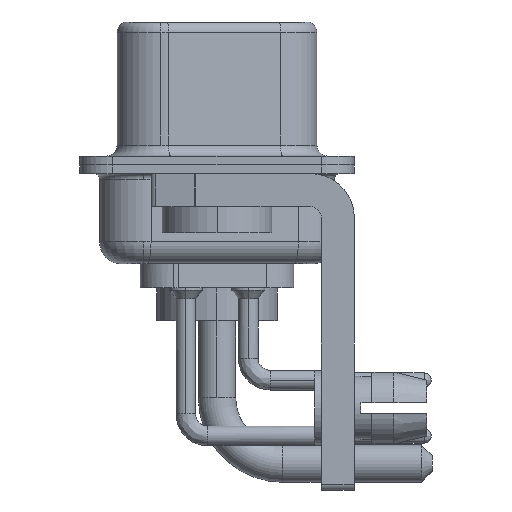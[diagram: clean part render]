
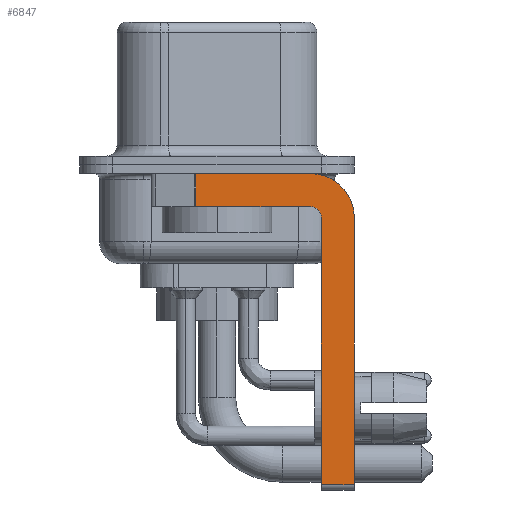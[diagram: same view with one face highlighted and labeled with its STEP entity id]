
A CAD part, left-side view. The second image highlights one B-rep face of the part: STEP entity #6847.
In plain terms, the highlighted planar face has unit normal (-1, 0, 0).
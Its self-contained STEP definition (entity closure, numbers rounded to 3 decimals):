
#1237 = CARTESIAN_POINT ( 'NONE',  ( -2.9, -4.25, -2.4 ) ) ;
#2401 = CIRCLE ( 'NONE', #5590, 2. ) ;
#2518 = VERTEX_POINT ( 'NONE', #2725 ) ;
#2519 = DIRECTION ( 'NONE',  ( 1., 0., 0. ) ) ;
#2725 = CARTESIAN_POINT ( 'NONE',  ( -2.9, -6.25, -14.55 ) ) ;
#2909 = CARTESIAN_POINT ( 'NONE',  ( -2.9, -4.75, -2.4 ) ) ;
#3019 = CARTESIAN_POINT ( 'NONE',  ( -2.9, -4.75, -14.8 ) ) ;
#3163 = ORIENTED_EDGE ( 'NONE', *, *, #10574, .F. ) ;
#3232 = EDGE_LOOP ( 'NONE', ( #4987, #20058, #3163, #21788, #18680, #17428, #16876, #21166 ) ) ;
#3481 = CARTESIAN_POINT ( 'NONE',  ( -2.9, -4.25, -2.4 ) ) ;
#4480 = VECTOR ( 'NONE', #5663, 1000. ) ;
#4587 = DIRECTION ( 'NONE',  ( 0., 0., -1. ) ) ;
#4697 = LINE ( 'NONE', #15106, #12434 ) ;
#4965 = CARTESIAN_POINT ( 'NONE',  ( -2.9, -6.25, -2.4 ) ) ;
#4987 = ORIENTED_EDGE ( 'NONE', *, *, #9422, .F. ) ;
#5192 = LINE ( 'NONE', #11982, #18535 ) ;
#5563 = VERTEX_POINT ( 'NONE', #15872 ) ;
#5590 = AXIS2_PLACEMENT_3D ( 'NONE', #3481, #11929, #20415 ) ;
#5663 = DIRECTION ( 'NONE',  ( 0., 0., -1. ) ) ;
#6539 = VECTOR ( 'NONE', #16546, 1000. ) ;
#6847 = ADVANCED_FACE ( 'NONE', ( #11187 ), #12530, .F. ) ;
#7184 = VERTEX_POINT ( 'NONE', #10415 ) ;
#7391 = AXIS2_PLACEMENT_3D ( 'NONE', #1237, #14770, #19745 ) ;
#8220 = VERTEX_POINT ( 'NONE', #19374 ) ;
#8953 = CARTESIAN_POINT ( 'NONE',  ( -2.9, 0.978, -1.9 ) ) ;
#9261 = CARTESIAN_POINT ( 'NONE',  ( -2.9, 3., -0.4 ) ) ;
#9422 = EDGE_CURVE ( 'NONE', #5563, #17456, #12898, .T. ) ;
#9888 = EDGE_CURVE ( 'NONE', #16541, #2518, #16301, .T. ) ;
#10415 = CARTESIAN_POINT ( 'NONE',  ( -2.9, -4.75, -14.55 ) ) ;
#10536 = VECTOR ( 'NONE', #11935, 1000. ) ;
#10550 = VECTOR ( 'NONE', #16099, 1000. ) ;
#10574 = EDGE_CURVE ( 'NONE', #8220, #13044, #18664, .T. ) ;
#11187 = FACE_OUTER_BOUND ( 'NONE', #3232, .T. ) ;
#11207 = CARTESIAN_POINT ( 'NONE',  ( -2.9, -6.25, -2.4 ) ) ;
#11294 = EDGE_CURVE ( 'NONE', #17456, #16541, #2401, .T. ) ;
#11659 = EDGE_CURVE ( 'NONE', #18870, #8220, #16226, .T. ) ;
#11929 = DIRECTION ( 'NONE',  ( 1., 0., 0. ) ) ;
#11935 = DIRECTION ( 'NONE',  ( 0., 1., 0. ) ) ;
#11982 = CARTESIAN_POINT ( 'NONE',  ( -2.9, -4.25, -14.55 ) ) ;
#12434 = VECTOR ( 'NONE', #4587, 1000. ) ;
#12530 = PLANE ( 'NONE',  #17651 ) ;
#12898 = LINE ( 'NONE', #9261, #10550 ) ;
#13044 = VERTEX_POINT ( 'NONE', #8953 ) ;
#13380 = CARTESIAN_POINT ( 'NONE',  ( -2.9, -4.25, -1.9 ) ) ;
#13950 = EDGE_CURVE ( 'NONE', #5563, #13044, #4697, .T. ) ;
#14770 = DIRECTION ( 'NONE',  ( -1., 0., 0. ) ) ;
#15106 = CARTESIAN_POINT ( 'NONE',  ( -2.9, 0.978, -1.9 ) ) ;
#15872 = CARTESIAN_POINT ( 'NONE',  ( -2.9, 0.978, -0.4 ) ) ;
#16099 = DIRECTION ( 'NONE',  ( 0., -1., 0. ) ) ;
#16128 = EDGE_CURVE ( 'NONE', #7184, #2518, #5192, .T. ) ;
#16226 = CIRCLE ( 'NONE', #7391, 0.5 ) ;
#16301 = LINE ( 'NONE', #11207, #4480 ) ;
#16541 = VERTEX_POINT ( 'NONE', #4965 ) ;
#16546 = DIRECTION ( 'NONE',  ( 0., 0., 1. ) ) ;
#16876 = ORIENTED_EDGE ( 'NONE', *, *, #9888, .F. ) ;
#17428 = ORIENTED_EDGE ( 'NONE', *, *, #16128, .T. ) ;
#17456 = VERTEX_POINT ( 'NONE', #21712 ) ;
#17481 = DIRECTION ( 'NONE',  ( 0., -1., 0. ) ) ;
#17651 = AXIS2_PLACEMENT_3D ( 'NONE', #17706, #2519, #17920 ) ;
#17706 = CARTESIAN_POINT ( 'NONE',  ( -2.9, -4.25, -2.4 ) ) ;
#17920 = DIRECTION ( 'NONE',  ( 0., 0., -1. ) ) ;
#18535 = VECTOR ( 'NONE', #17481, 1000. ) ;
#18664 = LINE ( 'NONE', #13380, #10536 ) ;
#18680 = ORIENTED_EDGE ( 'NONE', *, *, #18891, .F. ) ;
#18870 = VERTEX_POINT ( 'NONE', #2909 ) ;
#18891 = EDGE_CURVE ( 'NONE', #7184, #18870, #21741, .T. ) ;
#19374 = CARTESIAN_POINT ( 'NONE',  ( -2.9, -4.25, -1.9 ) ) ;
#19745 = DIRECTION ( 'NONE',  ( 0., 0., 1. ) ) ;
#20058 = ORIENTED_EDGE ( 'NONE', *, *, #13950, .T. ) ;
#20415 = DIRECTION ( 'NONE',  ( 0., 0., -1. ) ) ;
#21166 = ORIENTED_EDGE ( 'NONE', *, *, #11294, .F. ) ;
#21712 = CARTESIAN_POINT ( 'NONE',  ( -2.9, -4.25, -0.4 ) ) ;
#21741 = LINE ( 'NONE', #3019, #6539 ) ;
#21788 = ORIENTED_EDGE ( 'NONE', *, *, #11659, .F. ) ;
